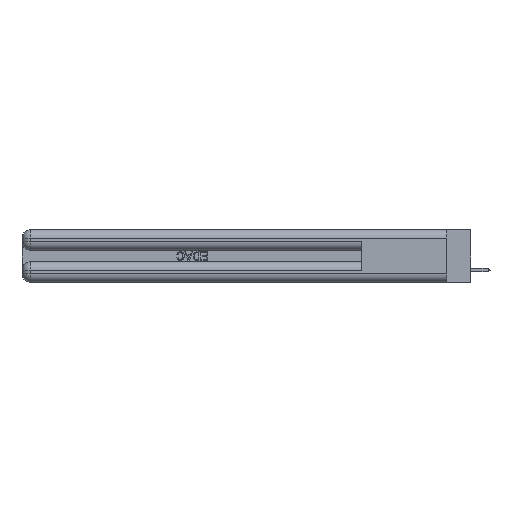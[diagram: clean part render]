
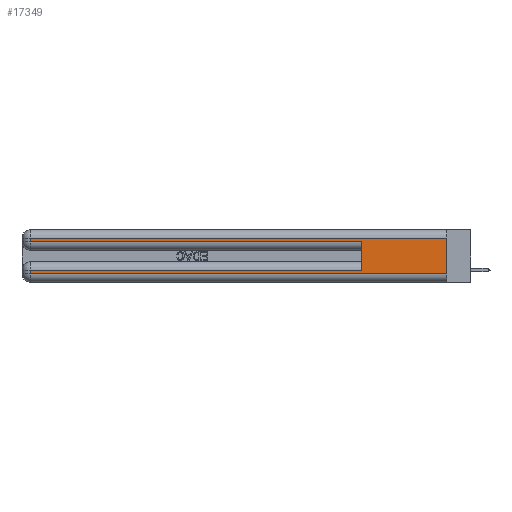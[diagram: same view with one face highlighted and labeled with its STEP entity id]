
A CAD part, left-side view. The second image highlights one B-rep face of the part: STEP entity #17349.
In plain terms, the highlighted planar face has unit normal (-1, 0, 0).
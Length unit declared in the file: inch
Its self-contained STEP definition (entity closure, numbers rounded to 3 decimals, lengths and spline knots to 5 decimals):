
#565 = VECTOR ( 'NONE', #13677, 39.37008 ) ;
#2382 = VECTOR ( 'NONE', #27617, 39.37008 ) ;
#3019 = VERTEX_POINT ( 'NONE', #6730 ) ;
#3625 = CARTESIAN_POINT ( 'NONE',  ( 0., 2.94, 0.37 ) ) ;
#4257 = LINE ( 'NONE', #28495, #8648 ) ;
#4301 = VECTOR ( 'NONE', #16351, 39.37008 ) ;
#4827 = CARTESIAN_POINT ( 'NONE',  ( 0., 0.6, 0.145 ) ) ;
#5257 = EDGE_CURVE ( 'NONE', #16583, #27057, #46273, .T. ) ;
#6730 = CARTESIAN_POINT ( 'NONE',  ( 0., 0., 0.06 ) ) ;
#6876 = CARTESIAN_POINT ( 'NONE',  ( 0., 2.94, 0.085 ) ) ;
#7521 = CARTESIAN_POINT ( 'NONE',  ( 0., 0., 0.37 ) ) ;
#8648 = VECTOR ( 'NONE', #27848, 39.37008 ) ;
#9733 = LINE ( 'NONE', #3625, #50419 ) ;
#10435 = PLANE ( 'NONE',  #44004 ) ;
#10974 = DIRECTION ( 'NONE',  ( 0., 0., -1. ) ) ;
#11352 = EDGE_CURVE ( 'NONE', #27057, #19214, #9733, .T. ) ;
#11768 = FACE_OUTER_BOUND ( 'NONE', #12431, .T. ) ;
#12431 = EDGE_LOOP ( 'NONE', ( #24553, #32435, #48234, #48646, #39272, #47861, #41410, #15095 ) ) ;
#12804 = CARTESIAN_POINT ( 'NONE',  ( 0., 0.6, 0.085 ) ) ;
#13141 = EDGE_CURVE ( 'NONE', #23572, #14665, #36539, .T. ) ;
#13414 = CARTESIAN_POINT ( 'NONE',  ( 0., 0., 0.085 ) ) ;
#13677 = DIRECTION ( 'NONE',  ( 0., 0., -1. ) ) ;
#13758 = VECTOR ( 'NONE', #47629, 39.37008 ) ;
#14665 = VERTEX_POINT ( 'NONE', #6876 ) ;
#15095 = ORIENTED_EDGE ( 'NONE', *, *, #43289, .T. ) ;
#15546 = CARTESIAN_POINT ( 'NONE',  ( 0., 2.94, 0.06 ) ) ;
#16351 = DIRECTION ( 'NONE',  ( 0., 0., 1. ) ) ;
#16583 = VERTEX_POINT ( 'NONE', #51709 ) ;
#17349 = ADVANCED_FACE ( 'NONE', ( #11768 ), #10435, .F. ) ;
#18652 = LINE ( 'NONE', #50719, #35527 ) ;
#18801 = CARTESIAN_POINT ( 'NONE',  ( 0., 0., 0.37 ) ) ;
#19214 = VERTEX_POINT ( 'NONE', #49826 ) ;
#21098 = CARTESIAN_POINT ( 'NONE',  ( 0., 2.94, 0.31 ) ) ;
#21993 = DIRECTION ( 'NONE',  ( 0., 1., 0. ) ) ;
#22052 = EDGE_CURVE ( 'NONE', #23572, #40696, #46833, .T. ) ;
#23572 = VERTEX_POINT ( 'NONE', #12804 ) ;
#23871 = CARTESIAN_POINT ( 'NONE',  ( 0., 0., 0.31 ) ) ;
#24553 = ORIENTED_EDGE ( 'NONE', *, *, #37783, .F. ) ;
#26199 = VERTEX_POINT ( 'NONE', #15546 ) ;
#27057 = VERTEX_POINT ( 'NONE', #21098 ) ;
#27617 = DIRECTION ( 'NONE',  ( 0., 0., -1. ) ) ;
#27848 = DIRECTION ( 'NONE',  ( 0., -1., 0. ) ) ;
#28055 = LINE ( 'NONE', #49771, #565 ) ;
#28495 = CARTESIAN_POINT ( 'NONE',  ( 0., 0., 0.285 ) ) ;
#29704 = EDGE_CURVE ( 'NONE', #14665, #26199, #28055, .T. ) ;
#32435 = ORIENTED_EDGE ( 'NONE', *, *, #5257, .T. ) ;
#33967 = EDGE_CURVE ( 'NONE', #19214, #40696, #4257, .T. ) ;
#35316 = VECTOR ( 'NONE', #21993, 39.37008 ) ;
#35527 = VECTOR ( 'NONE', #46824, 39.37008 ) ;
#36539 = LINE ( 'NONE', #13414, #35316 ) ;
#37783 = EDGE_CURVE ( 'NONE', #16583, #3019, #45454, .T. ) ;
#39272 = ORIENTED_EDGE ( 'NONE', *, *, #22052, .F. ) ;
#40696 = VERTEX_POINT ( 'NONE', #47754 ) ;
#41410 = ORIENTED_EDGE ( 'NONE', *, *, #29704, .T. ) ;
#43289 = EDGE_CURVE ( 'NONE', #26199, #3019, #18652, .T. ) ;
#43627 = DIRECTION ( 'NONE',  ( 0., 0., -1. ) ) ;
#44004 = AXIS2_PLACEMENT_3D ( 'NONE', #18801, #50861, #10974 ) ;
#45454 = LINE ( 'NONE', #7521, #2382 ) ;
#46273 = LINE ( 'NONE', #23871, #13758 ) ;
#46824 = DIRECTION ( 'NONE',  ( 0., -1., 0. ) ) ;
#46833 = LINE ( 'NONE', #4827, #4301 ) ;
#47629 = DIRECTION ( 'NONE',  ( 0., 1., 0. ) ) ;
#47754 = CARTESIAN_POINT ( 'NONE',  ( 0., 0.6, 0.285 ) ) ;
#47861 = ORIENTED_EDGE ( 'NONE', *, *, #13141, .T. ) ;
#48234 = ORIENTED_EDGE ( 'NONE', *, *, #11352, .T. ) ;
#48646 = ORIENTED_EDGE ( 'NONE', *, *, #33967, .T. ) ;
#49771 = CARTESIAN_POINT ( 'NONE',  ( 0., 2.94, 0.37 ) ) ;
#49826 = CARTESIAN_POINT ( 'NONE',  ( 0., 2.94, 0.285 ) ) ;
#50419 = VECTOR ( 'NONE', #43627, 39.37008 ) ;
#50719 = CARTESIAN_POINT ( 'NONE',  ( 0., 0., 0.06 ) ) ;
#50861 = DIRECTION ( 'NONE',  ( 1., 0., 0. ) ) ;
#51709 = CARTESIAN_POINT ( 'NONE',  ( 0., 0., 0.31 ) ) ;
